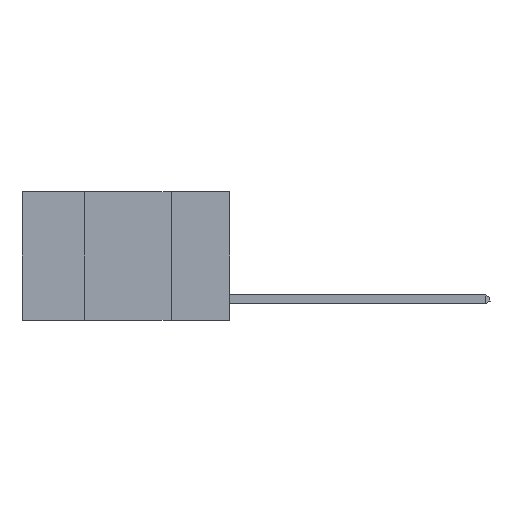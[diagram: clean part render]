
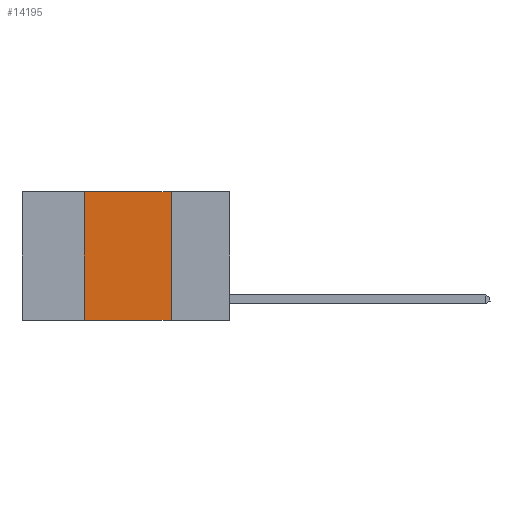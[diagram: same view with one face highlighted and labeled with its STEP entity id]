
A CAD part, left-side view. The second image highlights one B-rep face of the part: STEP entity #14195.
In plain terms, the highlighted planar face has unit normal (-1, 0, 0).
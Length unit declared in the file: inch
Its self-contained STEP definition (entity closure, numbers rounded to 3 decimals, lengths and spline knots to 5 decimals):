
#9 = EDGE_CURVE ( 'NONE', #4257, #11499, #2482, .T. ) ;
#83 = DIRECTION ( 'NONE',  ( 0., -1., 0. ) ) ;
#219 = FACE_OUTER_BOUND ( 'NONE', #12758, .T. ) ;
#420 = VECTOR ( 'NONE', #10230, 39.37008 ) ;
#1498 = CARTESIAN_POINT ( 'NONE',  ( 0., 0.42, 0. ) ) ;
#1626 = ORIENTED_EDGE ( 'NONE', *, *, #6553, .F. ) ;
#2482 = LINE ( 'NONE', #14469, #12019 ) ;
#2897 = CARTESIAN_POINT ( 'NONE',  ( 0., 0.17, 0. ) ) ;
#3405 = EDGE_CURVE ( 'NONE', #9191, #4257, #12913, .T. ) ;
#3883 = DIRECTION ( 'NONE',  ( 1., 0., 0. ) ) ;
#4257 = VERTEX_POINT ( 'NONE', #2897 ) ;
#5116 = LINE ( 'NONE', #7531, #11562 ) ;
#6449 = DIRECTION ( 'NONE',  ( 0., 0., -1. ) ) ;
#6553 = EDGE_CURVE ( 'NONE', #6810, #9191, #5116, .T. ) ;
#6617 = CARTESIAN_POINT ( 'NONE',  ( 0., 0.42, -0.37 ) ) ;
#6784 = CARTESIAN_POINT ( 'NONE',  ( 0., 0.17, -0.37 ) ) ;
#6810 = VERTEX_POINT ( 'NONE', #6617 ) ;
#6891 = ORIENTED_EDGE ( 'NONE', *, *, #10144, .T. ) ;
#7138 = CARTESIAN_POINT ( 'NONE',  ( 0., 0.6, 0. ) ) ;
#7531 = CARTESIAN_POINT ( 'NONE',  ( 0., 0.42, 0. ) ) ;
#7683 = ORIENTED_EDGE ( 'NONE', *, *, #9, .F. ) ;
#8189 = LINE ( 'NONE', #12697, #14270 ) ;
#8495 = DIRECTION ( 'NONE',  ( 0., 0., -1. ) ) ;
#9191 = VERTEX_POINT ( 'NONE', #1498 ) ;
#9726 = DIRECTION ( 'NONE',  ( 0., 0., 1. ) ) ;
#10051 = ORIENTED_EDGE ( 'NONE', *, *, #3405, .F. ) ;
#10144 = EDGE_CURVE ( 'NONE', #6810, #11499, #8189, .T. ) ;
#10230 = DIRECTION ( 'NONE',  ( 0., -1., 0. ) ) ;
#11499 = VERTEX_POINT ( 'NONE', #6784 ) ;
#11562 = VECTOR ( 'NONE', #9726, 39.37008 ) ;
#11882 = AXIS2_PLACEMENT_3D ( 'NONE', #14295, #3883, #8495 ) ;
#12019 = VECTOR ( 'NONE', #6449, 39.37008 ) ;
#12697 = CARTESIAN_POINT ( 'NONE',  ( 0., 0.6, -0.37 ) ) ;
#12758 = EDGE_LOOP ( 'NONE', ( #7683, #10051, #1626, #6891 ) ) ;
#12913 = LINE ( 'NONE', #7138, #420 ) ;
#14150 = PLANE ( 'NONE',  #11882 ) ;
#14195 = ADVANCED_FACE ( 'NONE', ( #219 ), #14150, .F. ) ;
#14270 = VECTOR ( 'NONE', #83, 39.37008 ) ;
#14295 = CARTESIAN_POINT ( 'NONE',  ( 0., 0.6, 0. ) ) ;
#14469 = CARTESIAN_POINT ( 'NONE',  ( 0., 0.17, 0. ) ) ;
